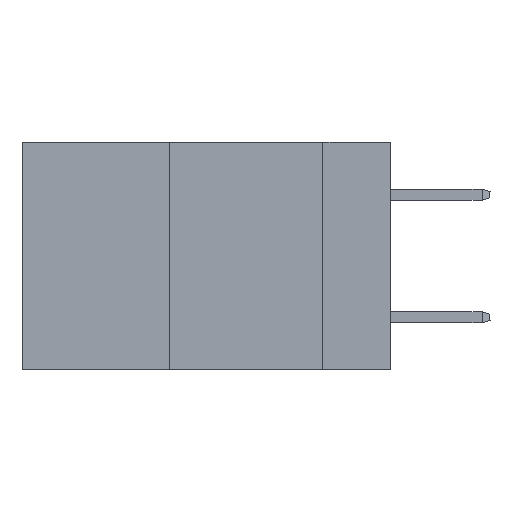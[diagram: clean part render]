
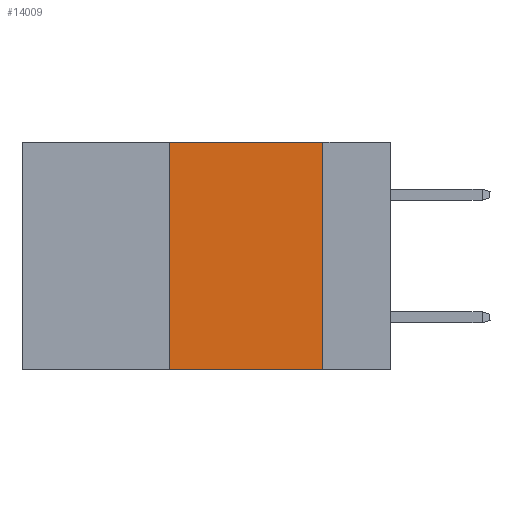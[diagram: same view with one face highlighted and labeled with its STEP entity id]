
A CAD part, left-side view. The second image highlights one B-rep face of the part: STEP entity #14009.
In plain terms, the highlighted planar face has unit normal (-1, 0, 0).
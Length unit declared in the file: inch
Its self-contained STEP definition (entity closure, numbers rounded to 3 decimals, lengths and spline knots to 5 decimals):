
#731 = DIRECTION ( 'NONE',  ( 1., 0., 0. ) ) ;
#979 = LINE ( 'NONE', #8983, #2115 ) ;
#1666 = VECTOR ( 'NONE', #17303, 39.37008 ) ;
#1976 = EDGE_CURVE ( 'NONE', #25601, #9074, #11157, .T. ) ;
#2115 = VECTOR ( 'NONE', #16063, 39.37008 ) ;
#2946 = DIRECTION ( 'NONE',  ( 0., 0., -1. ) ) ;
#3018 = VERTEX_POINT ( 'NONE', #7271 ) ;
#3062 = AXIS2_PLACEMENT_3D ( 'NONE', #5221, #731, #2946 ) ;
#5221 = CARTESIAN_POINT ( 'NONE',  ( 0., 0.6, 0. ) ) ;
#6309 = EDGE_CURVE ( 'NONE', #25601, #3018, #979, .T. ) ;
#6909 = ORIENTED_EDGE ( 'NONE', *, *, #6309, .T. ) ;
#7103 = ORIENTED_EDGE ( 'NONE', *, *, #8504, .F. ) ;
#7271 = CARTESIAN_POINT ( 'NONE',  ( 0., 0.11, -0.37 ) ) ;
#7648 = CARTESIAN_POINT ( 'NONE',  ( 0., 0.36, 0. ) ) ;
#7962 = LINE ( 'NONE', #8123, #1666 ) ;
#8123 = CARTESIAN_POINT ( 'NONE',  ( 0., 0.6, 0. ) ) ;
#8504 = EDGE_CURVE ( 'NONE', #9074, #9619, #7962, .T. ) ;
#8983 = CARTESIAN_POINT ( 'NONE',  ( 0., 0.6, -0.37 ) ) ;
#9074 = VERTEX_POINT ( 'NONE', #7648 ) ;
#9619 = VERTEX_POINT ( 'NONE', #12535 ) ;
#9987 = PLANE ( 'NONE',  #3062 ) ;
#11157 = LINE ( 'NONE', #19838, #28897 ) ;
#11376 = CARTESIAN_POINT ( 'NONE',  ( 0., 0.11, 0. ) ) ;
#12535 = CARTESIAN_POINT ( 'NONE',  ( 0., 0.11, 0. ) ) ;
#13982 = FACE_OUTER_BOUND ( 'NONE', #28635, .T. ) ;
#14009 = ADVANCED_FACE ( 'NONE', ( #13982 ), #9987, .F. ) ;
#14561 = EDGE_CURVE ( 'NONE', #9619, #3018, #15791, .T. ) ;
#15791 = LINE ( 'NONE', #11376, #25007 ) ;
#16063 = DIRECTION ( 'NONE',  ( 0., -1., 0. ) ) ;
#16920 = ORIENTED_EDGE ( 'NONE', *, *, #1976, .F. ) ;
#17303 = DIRECTION ( 'NONE',  ( 0., -1., 0. ) ) ;
#19838 = CARTESIAN_POINT ( 'NONE',  ( 0., 0.36, 0. ) ) ;
#21667 = DIRECTION ( 'NONE',  ( 0., 0., -1. ) ) ;
#24844 = CARTESIAN_POINT ( 'NONE',  ( 0., 0.36, -0.37 ) ) ;
#25007 = VECTOR ( 'NONE', #21667, 39.37008 ) ;
#25458 = ORIENTED_EDGE ( 'NONE', *, *, #14561, .F. ) ;
#25601 = VERTEX_POINT ( 'NONE', #24844 ) ;
#25696 = DIRECTION ( 'NONE',  ( 0., 0., 1. ) ) ;
#28635 = EDGE_LOOP ( 'NONE', ( #25458, #7103, #16920, #6909 ) ) ;
#28897 = VECTOR ( 'NONE', #25696, 39.37008 ) ;
